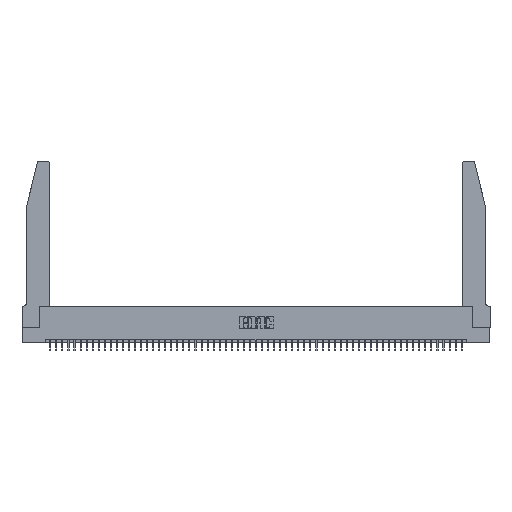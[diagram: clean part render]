
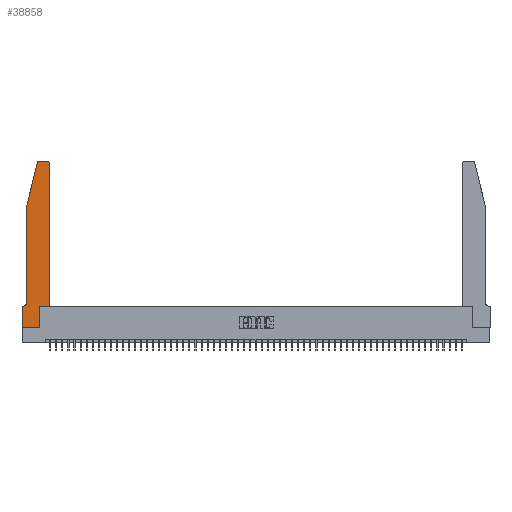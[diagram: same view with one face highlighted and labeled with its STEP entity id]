
A CAD part, top view. The second image highlights one B-rep face of the part: STEP entity #38858.
In plain terms, the highlighted planar face has unit normal (0, 0, 1).
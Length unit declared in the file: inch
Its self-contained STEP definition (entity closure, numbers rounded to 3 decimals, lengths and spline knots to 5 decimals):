
#32 = DIRECTION ( 'NONE',  ( 0., -1., 0. ) ) ;
#704 = EDGE_CURVE ( 'NONE', #35154, #22155, #51844, .T. ) ;
#1044 = LINE ( 'NONE', #34185, #49030 ) ;
#1854 = AXIS2_PLACEMENT_3D ( 'NONE', #6010, #40010, #53444 ) ;
#1885 = VERTEX_POINT ( 'NONE', #54345 ) ;
#2301 = CARTESIAN_POINT ( 'NONE',  ( 0.4505, 0.35, 0.37 ) ) ;
#2700 = CARTESIAN_POINT ( 'NONE',  ( 0.0055, 0.42, 0.37 ) ) ;
#4687 = ORIENTED_EDGE ( 'NONE', *, *, #27685, .T. ) ;
#5566 = DIRECTION ( 'NONE',  ( 0., 0., 1. ) ) ;
#5747 = CARTESIAN_POINT ( 'NONE',  ( 0.2865, 0.35, 0.37 ) ) ;
#6010 = CARTESIAN_POINT ( 'NONE',  ( 0.284, 2.72, 0.37 ) ) ;
#7238 = VERTEX_POINT ( 'NONE', #2301 ) ;
#7533 = EDGE_CURVE ( 'NONE', #1885, #41684, #31675, .T. ) ;
#8648 = ORIENTED_EDGE ( 'NONE', *, *, #7533, .T. ) ;
#9403 = CARTESIAN_POINT ( 'NONE',  ( 0.284, 2.75, 0.37 ) ) ;
#9498 = DIRECTION ( 'NONE',  ( 1., 0., 0. ) ) ;
#10003 = EDGE_CURVE ( 'NONE', #46327, #39986, #28527, .T. ) ;
#10539 = DIRECTION ( 'NONE',  ( 1., 0., 0. ) ) ;
#10721 = VERTEX_POINT ( 'NONE', #19962 ) ;
#10900 = CARTESIAN_POINT ( 'NONE',  ( 0.4505, 2.72, 0.37 ) ) ;
#11567 = DIRECTION ( 'NONE',  ( 0., 0., 1. ) ) ;
#12629 = ORIENTED_EDGE ( 'NONE', *, *, #50860, .T. ) ;
#13089 = DIRECTION ( 'NONE',  ( 1., 0., 0. ) ) ;
#13417 = CARTESIAN_POINT ( 'NONE',  ( 0.0755, 2., 0.37 ) ) ;
#13969 = DIRECTION ( 'NONE',  ( -0.239, -0.971, 0. ) ) ;
#15052 = CARTESIAN_POINT ( 'NONE',  ( 0.0755, 0.42, 0.37 ) ) ;
#15069 = CARTESIAN_POINT ( 'NONE',  ( 0.25487, 2.72718, 0.37 ) ) ;
#15671 = CARTESIAN_POINT ( 'NONE',  ( 0.0755, 0.35, 0.37 ) ) ;
#17552 = VECTOR ( 'NONE', #43772, 39.37008 ) ;
#17565 = VECTOR ( 'NONE', #32, 39.37008 ) ;
#17596 = VECTOR ( 'NONE', #10539, 39.37008 ) ;
#18991 = VECTOR ( 'NONE', #44314, 39.37008 ) ;
#19079 = EDGE_CURVE ( 'NONE', #41684, #35154, #50246, .T. ) ;
#19962 = CARTESIAN_POINT ( 'NONE',  ( 0.2865, 0., 0.37 ) ) ;
#20284 = VERTEX_POINT ( 'NONE', #5747 ) ;
#21658 = ORIENTED_EDGE ( 'NONE', *, *, #53498, .T. ) ;
#22155 = VERTEX_POINT ( 'NONE', #50045 ) ;
#22456 = LINE ( 'NONE', #35084, #17552 ) ;
#22887 = ORIENTED_EDGE ( 'NONE', *, *, #24032, .T. ) ;
#22956 = AXIS2_PLACEMENT_3D ( 'NONE', #2700, #54559, #41715 ) ;
#23230 = VERTEX_POINT ( 'NONE', #52875 ) ;
#24032 = EDGE_CURVE ( 'NONE', #7238, #53679, #25864, .T. ) ;
#24784 = FACE_OUTER_BOUND ( 'NONE', #25903, .T. ) ;
#25864 = LINE ( 'NONE', #48017, #46137 ) ;
#25903 = EDGE_LOOP ( 'NONE', ( #8648, #45248, #51231, #29149, #29735, #44523, #4687, #41588, #41819, #12629, #22887, #21658 ) ) ;
#26316 = VERTEX_POINT ( 'NONE', #15052 ) ;
#27348 = CARTESIAN_POINT ( 'NONE',  ( 0.0755, 2., 0.37 ) ) ;
#27685 = EDGE_CURVE ( 'NONE', #39986, #23230, #47156, .T. ) ;
#27917 = LINE ( 'NONE', #53485, #17596 ) ;
#28527 = LINE ( 'NONE', #15671, #30569 ) ;
#28671 = DIRECTION ( 'NONE',  ( 1., 0., 0. ) ) ;
#29149 = ORIENTED_EDGE ( 'NONE', *, *, #34220, .T. ) ;
#29735 = ORIENTED_EDGE ( 'NONE', *, *, #38372, .T. ) ;
#30569 = VECTOR ( 'NONE', #50441, 39.37008 ) ;
#31116 = CARTESIAN_POINT ( 'NONE',  ( 0.2605, 2.75, 0.37 ) ) ;
#31675 = LINE ( 'NONE', #31116, #18991 ) ;
#34185 = CARTESIAN_POINT ( 'NONE',  ( 0., 0., 0.37 ) ) ;
#34220 = EDGE_CURVE ( 'NONE', #22155, #26316, #47880, .T. ) ;
#35084 = CARTESIAN_POINT ( 'NONE',  ( 0.2865, 0.35, 0.37 ) ) ;
#35154 = VERTEX_POINT ( 'NONE', #15069 ) ;
#35525 = DIRECTION ( 'NONE',  ( 0., -1., 0. ) ) ;
#38372 = EDGE_CURVE ( 'NONE', #26316, #46327, #47158, .T. ) ;
#38467 = CARTESIAN_POINT ( 'NONE',  ( 0., 0., 0.37 ) ) ;
#38858 = ADVANCED_FACE ( 'NONE', ( #24784 ), #50028, .T. ) ;
#39078 = DIRECTION ( 'NONE',  ( 0., 1., 0. ) ) ;
#39986 = VERTEX_POINT ( 'NONE', #52649 ) ;
#40010 = DIRECTION ( 'NONE',  ( 0., 0., 1. ) ) ;
#41588 = ORIENTED_EDGE ( 'NONE', *, *, #51712, .T. ) ;
#41672 = VECTOR ( 'NONE', #35525, 39.37008 ) ;
#41684 = VERTEX_POINT ( 'NONE', #9403 ) ;
#41715 = DIRECTION ( 'NONE',  ( -1., 0., 0. ) ) ;
#41819 = ORIENTED_EDGE ( 'NONE', *, *, #50343, .T. ) ;
#41913 = CARTESIAN_POINT ( 'NONE',  ( 0., 0.35, 0.37 ) ) ;
#42759 = AXIS2_PLACEMENT_3D ( 'NONE', #41913, #11567, #28671 ) ;
#43772 = DIRECTION ( 'NONE',  ( 0., 1., 0. ) ) ;
#43797 = CIRCLE ( 'NONE', #48265, 0.03 ) ;
#44314 = DIRECTION ( 'NONE',  ( -1., 0., 0. ) ) ;
#44523 = ORIENTED_EDGE ( 'NONE', *, *, #10003, .T. ) ;
#44779 = VECTOR ( 'NONE', #13969, 39.37008 ) ;
#45248 = ORIENTED_EDGE ( 'NONE', *, *, #19079, .T. ) ;
#46137 = VECTOR ( 'NONE', #39078, 39.37008 ) ;
#46327 = VERTEX_POINT ( 'NONE', #47429 ) ;
#47156 = LINE ( 'NONE', #38467, #17565 ) ;
#47158 = CIRCLE ( 'NONE', #22956, 0.07 ) ;
#47429 = CARTESIAN_POINT ( 'NONE',  ( 0.0055, 0.35, 0.37 ) ) ;
#47880 = LINE ( 'NONE', #27348, #41672 ) ;
#48017 = CARTESIAN_POINT ( 'NONE',  ( 0.4505, 0.35, 0.37 ) ) ;
#48265 = AXIS2_PLACEMENT_3D ( 'NONE', #52145, #5566, #9498 ) ;
#49030 = VECTOR ( 'NONE', #13089, 39.37008 ) ;
#50028 = PLANE ( 'NONE',  #42759 ) ;
#50045 = CARTESIAN_POINT ( 'NONE',  ( 0.0755, 2., 0.37 ) ) ;
#50246 = CIRCLE ( 'NONE', #1854, 0.03 ) ;
#50343 = EDGE_CURVE ( 'NONE', #10721, #20284, #22456, .T. ) ;
#50441 = DIRECTION ( 'NONE',  ( -1., 0., 0. ) ) ;
#50860 = EDGE_CURVE ( 'NONE', #20284, #7238, #27917, .T. ) ;
#51231 = ORIENTED_EDGE ( 'NONE', *, *, #704, .T. ) ;
#51712 = EDGE_CURVE ( 'NONE', #23230, #10721, #1044, .T. ) ;
#51844 = LINE ( 'NONE', #13417, #44779 ) ;
#52145 = CARTESIAN_POINT ( 'NONE',  ( 0.4205, 2.72, 0.37 ) ) ;
#52649 = CARTESIAN_POINT ( 'NONE',  ( 0., 0.35, 0.37 ) ) ;
#52875 = CARTESIAN_POINT ( 'NONE',  ( 0., 0., 0.37 ) ) ;
#53444 = DIRECTION ( 'NONE',  ( 1., 0., 0. ) ) ;
#53485 = CARTESIAN_POINT ( 'NONE',  ( 0.4505, 0.35, 0.37 ) ) ;
#53498 = EDGE_CURVE ( 'NONE', #53679, #1885, #43797, .T. ) ;
#53679 = VERTEX_POINT ( 'NONE', #10900 ) ;
#54345 = CARTESIAN_POINT ( 'NONE',  ( 0.4205, 2.75, 0.37 ) ) ;
#54559 = DIRECTION ( 'NONE',  ( 0., 0., -1. ) ) ;
